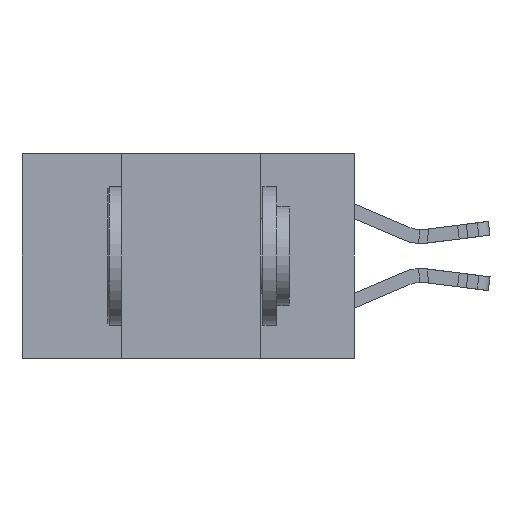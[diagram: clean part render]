
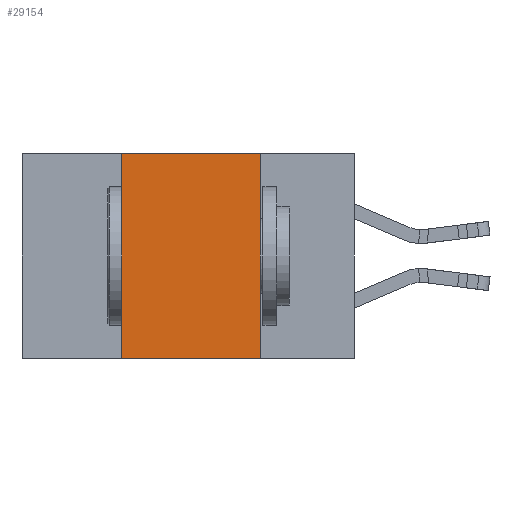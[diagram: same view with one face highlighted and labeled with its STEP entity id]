
A CAD part, left-side view. The second image highlights one B-rep face of the part: STEP entity #29154.
In plain terms, the highlighted planar face has unit normal (-1, 0, 0).
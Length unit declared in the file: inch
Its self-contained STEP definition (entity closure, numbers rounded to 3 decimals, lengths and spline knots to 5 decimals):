
#96 = AXIS2_PLACEMENT_3D ( 'NONE', #15334, #22801, #20310 ) ;
#190 = FACE_OUTER_BOUND ( 'NONE', #29174, .T. ) ;
#2283 = VERTEX_POINT ( 'NONE', #25176 ) ;
#2568 = DIRECTION ( 'NONE',  ( 0., -1., 0. ) ) ;
#2946 = LINE ( 'NONE', #29110, #25253 ) ;
#3566 = ORIENTED_EDGE ( 'NONE', *, *, #31997, .F. ) ;
#5226 = CARTESIAN_POINT ( 'NONE',  ( 0., 0.42, 0. ) ) ;
#6103 = VERTEX_POINT ( 'NONE', #9267 ) ;
#6394 = EDGE_CURVE ( 'NONE', #20337, #2283, #8855, .T. ) ;
#6789 = VECTOR ( 'NONE', #17897, 39.37008 ) ;
#7264 = VECTOR ( 'NONE', #29674, 39.37008 ) ;
#8176 = EDGE_CURVE ( 'NONE', #11199, #6103, #21284, .T. ) ;
#8199 = VECTOR ( 'NONE', #2568, 39.37008 ) ;
#8683 = CARTESIAN_POINT ( 'NONE',  ( 0., 0.17, 0. ) ) ;
#8855 = LINE ( 'NONE', #31994, #7264 ) ;
#8974 = DIRECTION ( 'NONE',  ( 0., -1., 0. ) ) ;
#9267 = CARTESIAN_POINT ( 'NONE',  ( 0., 0.42, 0. ) ) ;
#10048 = ORIENTED_EDGE ( 'NONE', *, *, #6394, .F. ) ;
#11199 = VERTEX_POINT ( 'NONE', #29429 ) ;
#11263 = ORIENTED_EDGE ( 'NONE', *, *, #22909, .T. ) ;
#14873 = CARTESIAN_POINT ( 'NONE',  ( 0., 0.6, 0. ) ) ;
#15334 = CARTESIAN_POINT ( 'NONE',  ( 0., 0.6, 0. ) ) ;
#15650 = PLANE ( 'NONE',  #96 ) ;
#17897 = DIRECTION ( 'NONE',  ( 0., 0., 1. ) ) ;
#20310 = DIRECTION ( 'NONE',  ( 0., 0., -1. ) ) ;
#20337 = VERTEX_POINT ( 'NONE', #8683 ) ;
#21284 = LINE ( 'NONE', #5226, #6789 ) ;
#22310 = LINE ( 'NONE', #14873, #8199 ) ;
#22801 = DIRECTION ( 'NONE',  ( 1., 0., 0. ) ) ;
#22909 = EDGE_CURVE ( 'NONE', #11199, #2283, #2946, .T. ) ;
#25176 = CARTESIAN_POINT ( 'NONE',  ( 0., 0.17, -0.37 ) ) ;
#25253 = VECTOR ( 'NONE', #8974, 39.37008 ) ;
#26402 = ORIENTED_EDGE ( 'NONE', *, *, #8176, .F. ) ;
#29110 = CARTESIAN_POINT ( 'NONE',  ( 0., 0.6, -0.37 ) ) ;
#29154 = ADVANCED_FACE ( 'NONE', ( #190 ), #15650, .F. ) ;
#29174 = EDGE_LOOP ( 'NONE', ( #10048, #3566, #26402, #11263 ) ) ;
#29429 = CARTESIAN_POINT ( 'NONE',  ( 0., 0.42, -0.37 ) ) ;
#29674 = DIRECTION ( 'NONE',  ( 0., 0., -1. ) ) ;
#31994 = CARTESIAN_POINT ( 'NONE',  ( 0., 0.17, 0. ) ) ;
#31997 = EDGE_CURVE ( 'NONE', #6103, #20337, #22310, .T. ) ;
